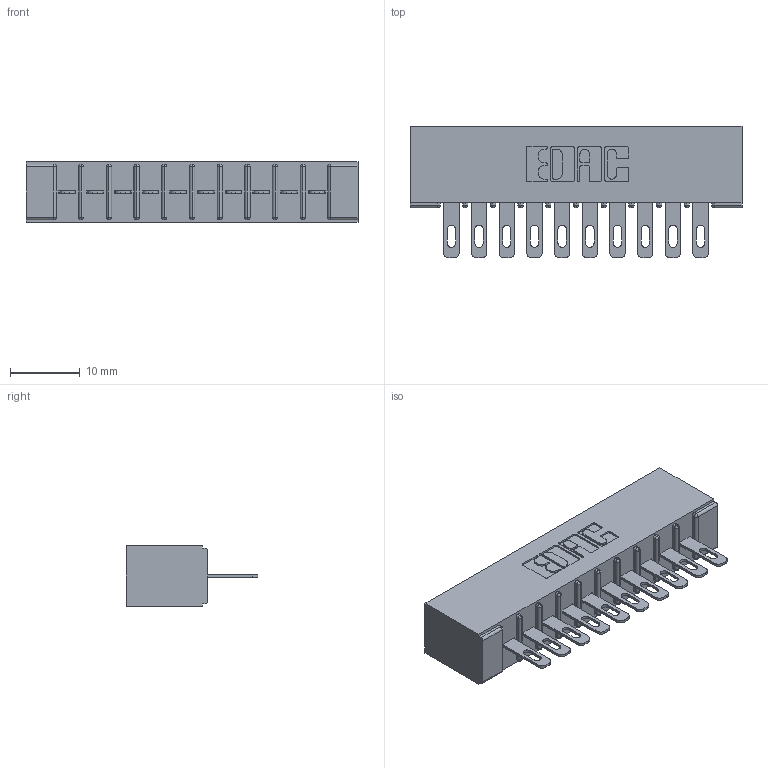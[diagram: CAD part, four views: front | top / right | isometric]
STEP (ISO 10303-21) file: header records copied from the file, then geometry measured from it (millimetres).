
FILE_DESCRIPTION (( 'STEP AP203' ), '1' );
FILE_NAME ('306-010-500-101.STEP', '2019-09-11T19:14:15', ( '' ), ( '' ), 'SwSTEP 2.0', 'SolidWorks 2016', '' );
FILE_SCHEMA (( 'CONFIG_CONTROL_DESIGN' ));
Length unit declared in the file: inch
Products named in the file (3): 306 Part_No Mounting; 306-290-001_100; 306-010-500-101
Assembly tree (11 placements, depth 2):
  306-010-500-101
    306 Part_No Mounting
    306-290-001_100  x10
Bounding box: 47.5 x 18.87 x 8.71 mm (x, y, z)
Volume: 3500.4 mm3; surface area: 5224.2 mm2
Topology: 11 solids, 11 shells, 868 faces, 2442 edges, 1572 vertices
Faces by surface type: plane 564, cylinder 264, sphere 40
Entity records: 13357 total; most frequent: CARTESIAN_POINT 2237, ORIENTED_EDGE 2212, DIRECTION 2210, EDGE_CURVE 1106, LINE 848, VECTOR 848, VERTEX_POINT 708, AXIS2_PLACEMENT_3D 681
